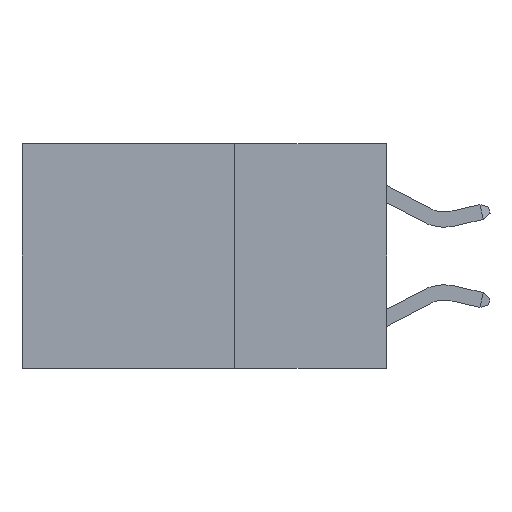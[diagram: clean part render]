
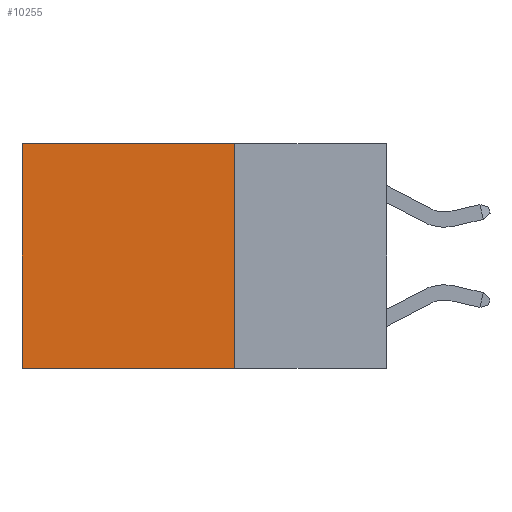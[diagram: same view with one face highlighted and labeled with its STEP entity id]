
A CAD part, left-side view. The second image highlights one B-rep face of the part: STEP entity #10255.
In plain terms, the highlighted planar face has unit normal (-1, 0, 0).
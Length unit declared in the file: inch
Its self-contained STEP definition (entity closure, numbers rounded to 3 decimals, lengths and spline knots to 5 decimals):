
#1833 = EDGE_CURVE ( 'NONE', #15781, #20886, #10905, .T. ) ;
#2221 = EDGE_CURVE ( 'NONE', #15781, #2468, #16269, .T. ) ;
#2468 = VERTEX_POINT ( 'NONE', #18757 ) ;
#3714 = CARTESIAN_POINT ( 'NONE',  ( 0.2625, 0.6, 0. ) ) ;
#7290 = FACE_OUTER_BOUND ( 'NONE', #9943, .T. ) ;
#7896 = LINE ( 'NONE', #15095, #12057 ) ;
#8215 = EDGE_CURVE ( 'NONE', #2468, #20924, #7896, .T. ) ;
#8920 = ORIENTED_EDGE ( 'NONE', *, *, #1833, .T. ) ;
#9325 = CARTESIAN_POINT ( 'NONE',  ( 0.2625, 0.25, 0. ) ) ;
#9727 = DIRECTION ( 'NONE',  ( 0., 1., 0. ) ) ;
#9943 = EDGE_LOOP ( 'NONE', ( #20436, #15483, #11007, #8920 ) ) ;
#10255 = ADVANCED_FACE ( 'NONE', ( #7290 ), #20126, .F. ) ;
#10905 = LINE ( 'NONE', #20520, #15718 ) ;
#11007 = ORIENTED_EDGE ( 'NONE', *, *, #2221, .F. ) ;
#11133 = DIRECTION ( 'NONE',  ( 0., 0., -1. ) ) ;
#12057 = VECTOR ( 'NONE', #16924, 39.37008 ) ;
#12770 = LINE ( 'NONE', #3714, #21747 ) ;
#14508 = DIRECTION ( 'NONE',  ( 0., 0., -1. ) ) ;
#14746 = AXIS2_PLACEMENT_3D ( 'NONE', #9325, #21887, #11133 ) ;
#15095 = CARTESIAN_POINT ( 'NONE',  ( 0.2625, 0.25, -0.37 ) ) ;
#15483 = ORIENTED_EDGE ( 'NONE', *, *, #8215, .F. ) ;
#15718 = VECTOR ( 'NONE', #9727, 39.37008 ) ;
#15781 = VERTEX_POINT ( 'NONE', #20677 ) ;
#16269 = LINE ( 'NONE', #19869, #20479 ) ;
#16837 = CARTESIAN_POINT ( 'NONE',  ( 0.2625, 0.6, 0. ) ) ;
#16924 = DIRECTION ( 'NONE',  ( 0., 1., 0. ) ) ;
#18090 = DIRECTION ( 'NONE',  ( 0., 0., -1. ) ) ;
#18757 = CARTESIAN_POINT ( 'NONE',  ( 0.2625, 0.25, -0.37 ) ) ;
#18764 = CARTESIAN_POINT ( 'NONE',  ( 0.2625, 0.6, -0.37 ) ) ;
#19869 = CARTESIAN_POINT ( 'NONE',  ( 0.2625, 0.25, 0. ) ) ;
#20126 = PLANE ( 'NONE',  #14746 ) ;
#20436 = ORIENTED_EDGE ( 'NONE', *, *, #22492, .T. ) ;
#20479 = VECTOR ( 'NONE', #14508, 39.37008 ) ;
#20520 = CARTESIAN_POINT ( 'NONE',  ( 0.2625, 0.25, 0. ) ) ;
#20677 = CARTESIAN_POINT ( 'NONE',  ( 0.2625, 0.25, 0. ) ) ;
#20886 = VERTEX_POINT ( 'NONE', #16837 ) ;
#20924 = VERTEX_POINT ( 'NONE', #18764 ) ;
#21747 = VECTOR ( 'NONE', #18090, 39.37008 ) ;
#21887 = DIRECTION ( 'NONE',  ( 1., 0., 0. ) ) ;
#22492 = EDGE_CURVE ( 'NONE', #20886, #20924, #12770, .T. ) ;
